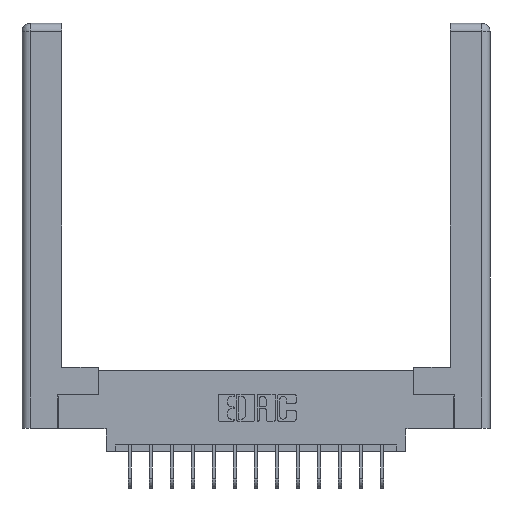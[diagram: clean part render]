
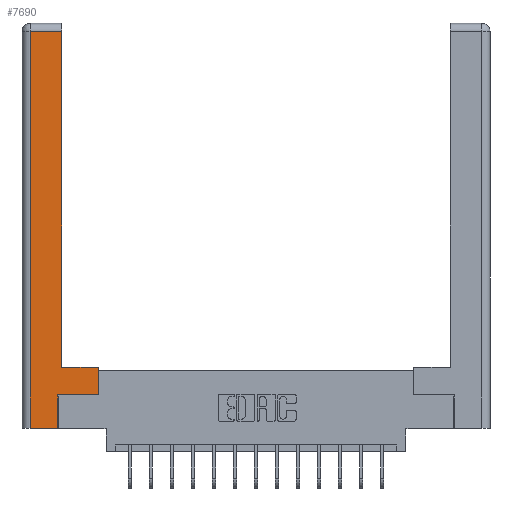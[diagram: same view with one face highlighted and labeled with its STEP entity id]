
A CAD part, top view. The second image highlights one B-rep face of the part: STEP entity #7690.
In plain terms, the highlighted planar face has unit normal (0, 0, 1).
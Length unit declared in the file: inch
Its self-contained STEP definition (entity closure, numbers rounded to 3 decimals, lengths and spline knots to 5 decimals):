
#573 = ORIENTED_EDGE ( 'NONE', *, *, #3509, .T. ) ;
#583 = EDGE_CURVE ( 'NONE', #15118, #6660, #12876, .T. ) ;
#635 = LINE ( 'NONE', #13158, #5968 ) ;
#837 = VECTOR ( 'NONE', #14245, 39.37008 ) ;
#868 = VECTOR ( 'NONE', #8250, 39.37008 ) ;
#1144 = VERTEX_POINT ( 'NONE', #13112 ) ;
#1174 = CARTESIAN_POINT ( 'NONE',  ( 0.295, 3., 0. ) ) ;
#1201 = CARTESIAN_POINT ( 'NONE',  ( 0.565, 0.245, 0. ) ) ;
#1333 = DIRECTION ( 'NONE',  ( 0., 0., -1. ) ) ;
#1380 = FACE_OUTER_BOUND ( 'NONE', #14985, .T. ) ;
#1391 = CARTESIAN_POINT ( 'NONE',  ( 0.565, 0.45, 0. ) ) ;
#1500 = CARTESIAN_POINT ( 'NONE',  ( 0., 0., 0. ) ) ;
#1570 = CARTESIAN_POINT ( 'NONE',  ( 0.295, 0.45, 0. ) ) ;
#1651 = LINE ( 'NONE', #1570, #837 ) ;
#1815 = LINE ( 'NONE', #14767, #12820 ) ;
#2438 = VERTEX_POINT ( 'NONE', #5556 ) ;
#2701 = VERTEX_POINT ( 'NONE', #3578 ) ;
#2895 = LINE ( 'NONE', #1174, #6229 ) ;
#3377 = VECTOR ( 'NONE', #5324, 39.37008 ) ;
#3509 = EDGE_CURVE ( 'NONE', #2701, #15118, #9519, .T. ) ;
#3578 = CARTESIAN_POINT ( 'NONE',  ( 0.265, 0., 0. ) ) ;
#3911 = DIRECTION ( 'NONE',  ( -1., 0., 0. ) ) ;
#4710 = EDGE_CURVE ( 'NONE', #12761, #2701, #635, .T. ) ;
#5324 = DIRECTION ( 'NONE',  ( 0., 1., 0. ) ) ;
#5403 = CARTESIAN_POINT ( 'NONE',  ( 0.265, 0.245, 0. ) ) ;
#5556 = CARTESIAN_POINT ( 'NONE',  ( 0.0615, 2.94, 0. ) ) ;
#5968 = VECTOR ( 'NONE', #6913, 39.37008 ) ;
#6229 = VECTOR ( 'NONE', #9892, 39.37008 ) ;
#6257 = ORIENTED_EDGE ( 'NONE', *, *, #14528, .T. ) ;
#6352 = VECTOR ( 'NONE', #13666, 39.37008 ) ;
#6572 = CARTESIAN_POINT ( 'NONE',  ( 0.295, 0.45, 0. ) ) ;
#6660 = VERTEX_POINT ( 'NONE', #14201 ) ;
#6895 = CARTESIAN_POINT ( 'NONE',  ( 0.265, 0.245, 0. ) ) ;
#6913 = DIRECTION ( 'NONE',  ( 1., 0., 0. ) ) ;
#7164 = LINE ( 'NONE', #15297, #13862 ) ;
#7690 = ADVANCED_FACE ( 'NONE', ( #1380 ), #8985, .F. ) ;
#7924 = CARTESIAN_POINT ( 'NONE',  ( 0.0615, 0., 0. ) ) ;
#8250 = DIRECTION ( 'NONE',  ( 0., 1., 0. ) ) ;
#8472 = DIRECTION ( 'NONE',  ( 0., -1., 0. ) ) ;
#8553 = ORIENTED_EDGE ( 'NONE', *, *, #583, .T. ) ;
#8985 = PLANE ( 'NONE',  #12393 ) ;
#9037 = LINE ( 'NONE', #15307, #3377 ) ;
#9519 = LINE ( 'NONE', #6895, #868 ) ;
#9776 = VERTEX_POINT ( 'NONE', #6572 ) ;
#9892 = DIRECTION ( 'NONE',  ( 0., 1., 0. ) ) ;
#10219 = VERTEX_POINT ( 'NONE', #1391 ) ;
#10274 = DIRECTION ( 'NONE',  ( -1., 0., 0. ) ) ;
#10731 = EDGE_CURVE ( 'NONE', #2438, #12761, #1815, .T. ) ;
#12013 = EDGE_CURVE ( 'NONE', #6660, #10219, #9037, .T. ) ;
#12211 = ORIENTED_EDGE ( 'NONE', *, *, #4710, .T. ) ;
#12393 = AXIS2_PLACEMENT_3D ( 'NONE', #1500, #1333, #10274 ) ;
#12482 = EDGE_CURVE ( 'NONE', #9776, #1144, #2895, .T. ) ;
#12761 = VERTEX_POINT ( 'NONE', #7924 ) ;
#12820 = VECTOR ( 'NONE', #8472, 39.37008 ) ;
#12876 = LINE ( 'NONE', #1201, #6352 ) ;
#13112 = CARTESIAN_POINT ( 'NONE',  ( 0.295, 2.94, 0. ) ) ;
#13117 = EDGE_CURVE ( 'NONE', #1144, #2438, #7164, .T. ) ;
#13158 = CARTESIAN_POINT ( 'NONE',  ( 0.265, 0., 0. ) ) ;
#13241 = ORIENTED_EDGE ( 'NONE', *, *, #12013, .T. ) ;
#13615 = ORIENTED_EDGE ( 'NONE', *, *, #12482, .T. ) ;
#13666 = DIRECTION ( 'NONE',  ( 1., 0., 0. ) ) ;
#13862 = VECTOR ( 'NONE', #3911, 39.37008 ) ;
#14201 = CARTESIAN_POINT ( 'NONE',  ( 0.565, 0.245, 0. ) ) ;
#14245 = DIRECTION ( 'NONE',  ( -1., 0., 0. ) ) ;
#14528 = EDGE_CURVE ( 'NONE', #10219, #9776, #1651, .T. ) ;
#14767 = CARTESIAN_POINT ( 'NONE',  ( 0.0615, 0., 0. ) ) ;
#14985 = EDGE_LOOP ( 'NONE', ( #13615, #15445, #15828, #12211, #573, #8553, #13241, #6257 ) ) ;
#15118 = VERTEX_POINT ( 'NONE', #5403 ) ;
#15297 = CARTESIAN_POINT ( 'NONE',  ( 0.0615, 2.94, 0. ) ) ;
#15307 = CARTESIAN_POINT ( 'NONE',  ( 0.565, 0.45, 0. ) ) ;
#15445 = ORIENTED_EDGE ( 'NONE', *, *, #13117, .T. ) ;
#15828 = ORIENTED_EDGE ( 'NONE', *, *, #10731, .T. ) ;
